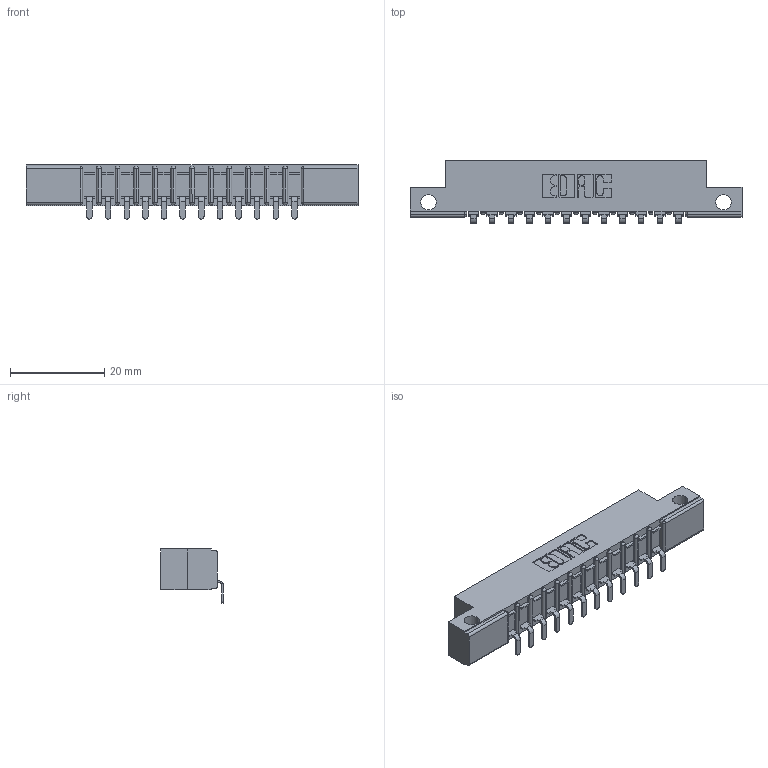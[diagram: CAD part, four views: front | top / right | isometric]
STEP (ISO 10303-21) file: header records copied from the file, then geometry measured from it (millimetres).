
FILE_DESCRIPTION (( 'STEP AP203' ), '1' );
FILE_NAME ('357-012-553-112.STEP', '2019-09-16T19:16:51', ( '' ), ( '' ), 'SwSTEP 2.0', 'SolidWorks 2016', '' );
FILE_SCHEMA (( 'CONFIG_CONTROL_DESIGN' ));
Length unit declared in the file: inch
Products named in the file (3): 357-012-553-112; 307 Part_.128 Dia Side Mounting Holes; 307-290-002_553
Assembly tree (13 placements, depth 2):
  357-012-553-112
    307 Part_.128 Dia Side Mounting Holes
    307-290-002_553  x12
Bounding box: 70.56 x 13.32 x 11.51 mm (x, y, z)
Volume: 4577.1 mm3; surface area: 7635 mm2
Topology: 13 solids, 13 shells, 1067 faces, 3251 edges, 2130 vertices
Faces by surface type: plane 634, cylinder 407, sphere 26
Entity records: 14842 total; most frequent: CARTESIAN_POINT 2500, ORIENTED_EDGE 2490, DIRECTION 2443, EDGE_CURVE 1245, LINE 937, VECTOR 937, VERTEX_POINT 810, AXIS2_PLACEMENT_3D 753
